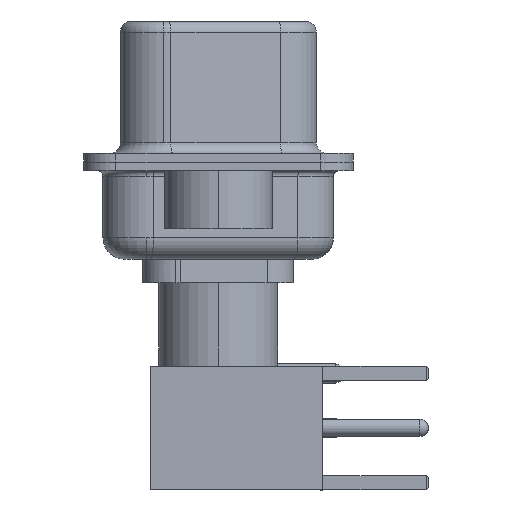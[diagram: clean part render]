
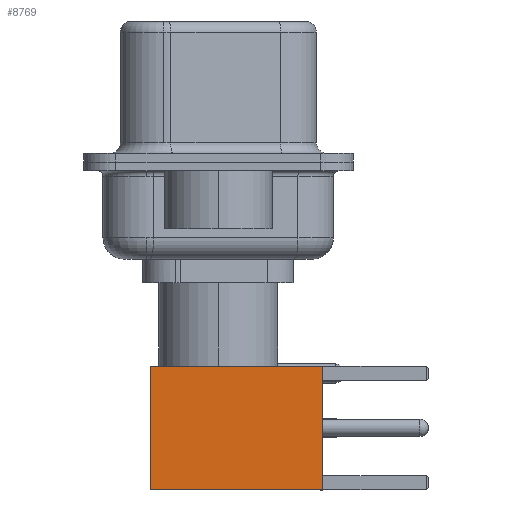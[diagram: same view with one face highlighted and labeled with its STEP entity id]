
A CAD part, left-side view. The second image highlights one B-rep face of the part: STEP entity #8769.
In plain terms, the highlighted face is planar.
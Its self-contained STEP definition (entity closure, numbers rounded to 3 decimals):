
#606 = DIRECTION ( 'NONE',  ( -1., 0., 0. ) ) ;
#1427 = DIRECTION ( 'NONE',  ( 0., 0., -1. ) ) ;
#2251 = DIRECTION ( 'NONE',  ( 0., 1., 0. ) ) ;
#3073 = VECTOR ( 'NONE', #25342, 1000. ) ;
#3239 = EDGE_CURVE ( 'NONE', #11239, #19261, #10573, .T. ) ;
#4155 = CARTESIAN_POINT ( 'NONE',  ( 2.875, 2.875, 8. ) ) ;
#6753 = ORIENTED_EDGE ( 'NONE', *, *, #3239, .T. ) ;
#7368 = VERTEX_POINT ( 'NONE', #23311 ) ;
#8769 = ADVANCED_FACE ( 'NONE', ( #19717 ), #21265, .T. ) ;
#9323 = ORIENTED_EDGE ( 'NONE', *, *, #12317, .T. ) ;
#9714 = LINE ( 'NONE', #18193, #3073 ) ;
#9928 = ORIENTED_EDGE ( 'NONE', *, *, #16065, .F. ) ;
#10573 = LINE ( 'NONE', #24832, #21222 ) ;
#11239 = VERTEX_POINT ( 'NONE', #4155 ) ;
#11620 = ORIENTED_EDGE ( 'NONE', *, *, #13903, .F. ) ;
#12317 = EDGE_CURVE ( 'NONE', #19261, #22948, #19343, .T. ) ;
#13638 = VECTOR ( 'NONE', #606, 1000. ) ;
#13712 = EDGE_LOOP ( 'NONE', ( #6753, #9323, #11620, #9928 ) ) ;
#13903 = EDGE_CURVE ( 'NONE', #7368, #22948, #20302, .T. ) ;
#15014 = CARTESIAN_POINT ( 'NONE',  ( 2.875, 2.875, 0. ) ) ;
#15290 = DIRECTION ( 'NONE',  ( 0., 0., 1. ) ) ;
#16065 = EDGE_CURVE ( 'NONE', #11239, #7368, #9714, .T. ) ;
#17957 = CARTESIAN_POINT ( 'NONE',  ( 2.875, 2.875, 0. ) ) ;
#18193 = CARTESIAN_POINT ( 'NONE',  ( 0., 2.875, 8. ) ) ;
#19261 = VERTEX_POINT ( 'NONE', #17957 ) ;
#19343 = LINE ( 'NONE', #19604, #13638 ) ;
#19604 = CARTESIAN_POINT ( 'NONE',  ( 0., 2.875, 0. ) ) ;
#19717 = FACE_OUTER_BOUND ( 'NONE', #13712, .T. ) ;
#20302 = LINE ( 'NONE', #20438, #23871 ) ;
#20438 = CARTESIAN_POINT ( 'NONE',  ( -2.875, 2.875, 0. ) ) ;
#21222 = VECTOR ( 'NONE', #25249, 1000. ) ;
#21265 = PLANE ( 'NONE',  #23110 ) ;
#22948 = VERTEX_POINT ( 'NONE', #23164 ) ;
#23110 = AXIS2_PLACEMENT_3D ( 'NONE', #15014, #2251, #15290 ) ;
#23164 = CARTESIAN_POINT ( 'NONE',  ( -2.875, 2.875, 0. ) ) ;
#23311 = CARTESIAN_POINT ( 'NONE',  ( -2.875, 2.875, 8. ) ) ;
#23871 = VECTOR ( 'NONE', #1427, 1000. ) ;
#24832 = CARTESIAN_POINT ( 'NONE',  ( 2.875, 2.875, 0. ) ) ;
#25249 = DIRECTION ( 'NONE',  ( 0., 0., -1. ) ) ;
#25342 = DIRECTION ( 'NONE',  ( -1., 0., 0. ) ) ;
